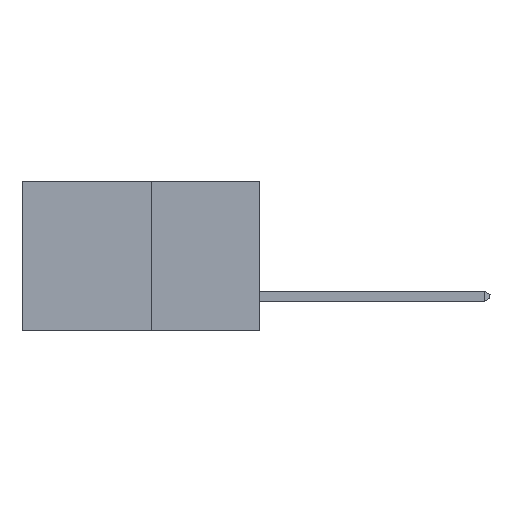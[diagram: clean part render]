
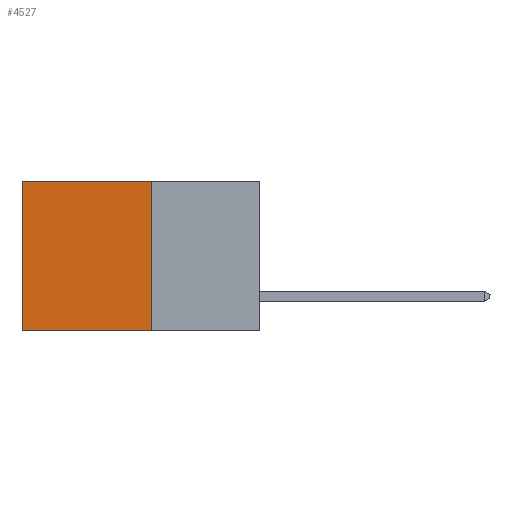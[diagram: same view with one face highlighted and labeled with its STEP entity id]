
A CAD part, left-side view. The second image highlights one B-rep face of the part: STEP entity #4527.
In plain terms, the highlighted planar face has unit normal (-1, 0, 0).
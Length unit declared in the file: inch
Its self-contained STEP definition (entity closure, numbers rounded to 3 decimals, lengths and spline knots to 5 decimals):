
#605 = EDGE_CURVE ( 'NONE', #18184, #11609, #12894, .T. ) ;
#1003 = EDGE_LOOP ( 'NONE', ( #16907, #9167, #1048, #2542 ) ) ;
#1048 = ORIENTED_EDGE ( 'NONE', *, *, #20175, .F. ) ;
#2542 = ORIENTED_EDGE ( 'NONE', *, *, #23745, .T. ) ;
#4492 = DIRECTION ( 'NONE',  ( 0., 0., -1. ) ) ;
#4527 = ADVANCED_FACE ( 'NONE', ( #20720 ), #22808, .F. ) ;
#4884 = LINE ( 'NONE', #7862, #9273 ) ;
#6304 = VECTOR ( 'NONE', #12230, 39.37008 ) ;
#6573 = CARTESIAN_POINT ( 'NONE',  ( 0.277, 0.27, 0. ) ) ;
#6896 = LINE ( 'NONE', #6573, #6304 ) ;
#7862 = CARTESIAN_POINT ( 'NONE',  ( 0.277, 0.59, -0.37 ) ) ;
#9167 = ORIENTED_EDGE ( 'NONE', *, *, #605, .F. ) ;
#9273 = VECTOR ( 'NONE', #22485, 39.37008 ) ;
#9999 = DIRECTION ( 'NONE',  ( 0., 0., -1. ) ) ;
#10841 = LINE ( 'NONE', #19150, #20575 ) ;
#11471 = CARTESIAN_POINT ( 'NONE',  ( 0.277, 0.59, -0.37 ) ) ;
#11510 = CARTESIAN_POINT ( 'NONE',  ( 0.277, 0.27, 0. ) ) ;
#11609 = VERTEX_POINT ( 'NONE', #11471 ) ;
#12230 = DIRECTION ( 'NONE',  ( 0., 1., 0. ) ) ;
#12307 = VECTOR ( 'NONE', #20495, 39.37008 ) ;
#12893 = AXIS2_PLACEMENT_3D ( 'NONE', #22729, #15583, #4492 ) ;
#12894 = LINE ( 'NONE', #20464, #12307 ) ;
#12918 = EDGE_CURVE ( 'NONE', #21665, #11609, #4884, .T. ) ;
#14893 = CARTESIAN_POINT ( 'NONE',  ( 0.277, 0.27, -0.37 ) ) ;
#15583 = DIRECTION ( 'NONE',  ( 1., 0., 0. ) ) ;
#16907 = ORIENTED_EDGE ( 'NONE', *, *, #12918, .T. ) ;
#18184 = VERTEX_POINT ( 'NONE', #14893 ) ;
#18288 = VERTEX_POINT ( 'NONE', #11510 ) ;
#19150 = CARTESIAN_POINT ( 'NONE',  ( 0.277, 0.27, -0.37 ) ) ;
#20175 = EDGE_CURVE ( 'NONE', #18288, #18184, #10841, .T. ) ;
#20464 = CARTESIAN_POINT ( 'NONE',  ( 0.277, 0.27, -0.37 ) ) ;
#20495 = DIRECTION ( 'NONE',  ( 0., 1., 0. ) ) ;
#20575 = VECTOR ( 'NONE', #9999, 39.37008 ) ;
#20720 = FACE_OUTER_BOUND ( 'NONE', #1003, .T. ) ;
#21665 = VERTEX_POINT ( 'NONE', #22446 ) ;
#22446 = CARTESIAN_POINT ( 'NONE',  ( 0.277, 0.59, 0. ) ) ;
#22485 = DIRECTION ( 'NONE',  ( 0., 0., -1. ) ) ;
#22729 = CARTESIAN_POINT ( 'NONE',  ( 0.277, 0.27, -0.37 ) ) ;
#22808 = PLANE ( 'NONE',  #12893 ) ;
#23745 = EDGE_CURVE ( 'NONE', #18288, #21665, #6896, .T. ) ;
